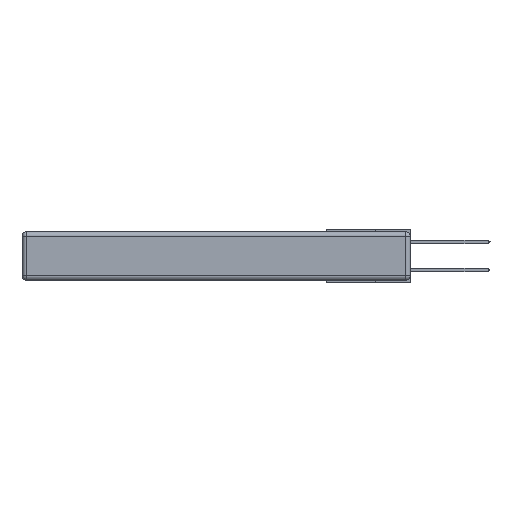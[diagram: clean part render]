
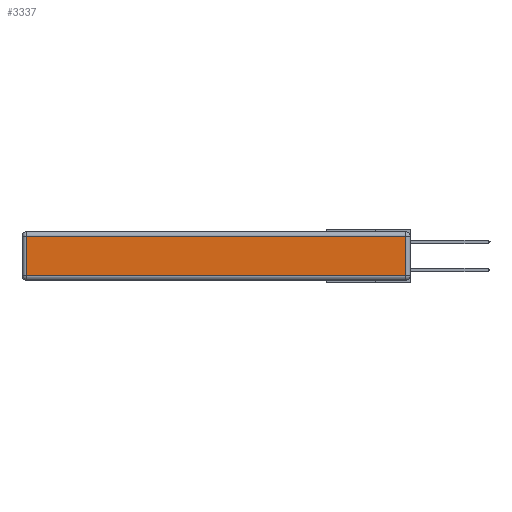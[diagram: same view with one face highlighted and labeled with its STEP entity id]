
A CAD part, left-side view. The second image highlights one B-rep face of the part: STEP entity #3337.
In plain terms, the highlighted planar face has unit normal (-1, 0, 0).
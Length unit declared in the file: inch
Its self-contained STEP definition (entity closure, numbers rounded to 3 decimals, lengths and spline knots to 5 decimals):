
#512 = VECTOR ( 'NONE', #9564, 39.37008 ) ;
#1010 = ORIENTED_EDGE ( 'NONE', *, *, #21946, .T. ) ;
#1089 = EDGE_CURVE ( 'NONE', #18587, #13305, #20870, .T. ) ;
#1495 = PLANE ( 'NONE',  #15933 ) ;
#1499 = DIRECTION ( 'NONE',  ( 0., 0., -1. ) ) ;
#2366 = CARTESIAN_POINT ( 'NONE',  ( 0., 2.75, -0.03 ) ) ;
#3337 = ADVANCED_FACE ( 'NONE', ( #21663 ), #1495, .T. ) ;
#3548 = DIRECTION ( 'NONE',  ( -1., 0., 0. ) ) ;
#3764 = ORIENTED_EDGE ( 'NONE', *, *, #1089, .T. ) ;
#4328 = CARTESIAN_POINT ( 'NONE',  ( 0., 0.03, -0.343 ) ) ;
#5006 = VERTEX_POINT ( 'NONE', #21774 ) ;
#8549 = VECTOR ( 'NONE', #8714, 39.37008 ) ;
#8714 = DIRECTION ( 'NONE',  ( 0., 1., 0. ) ) ;
#9564 = DIRECTION ( 'NONE',  ( 0., -1., 0. ) ) ;
#10054 = LINE ( 'NONE', #4328, #18641 ) ;
#10181 = EDGE_LOOP ( 'NONE', ( #3764, #17243, #1010, #20148 ) ) ;
#11650 = VECTOR ( 'NONE', #1499, 39.37008 ) ;
#13305 = VERTEX_POINT ( 'NONE', #22958 ) ;
#15309 = VERTEX_POINT ( 'NONE', #18770 ) ;
#15757 = CARTESIAN_POINT ( 'NONE',  ( 0., 0., -0.343 ) ) ;
#15778 = CARTESIAN_POINT ( 'NONE',  ( 0., 0., -0.313 ) ) ;
#15933 = AXIS2_PLACEMENT_3D ( 'NONE', #15757, #3548, #17799 ) ;
#16282 = EDGE_CURVE ( 'NONE', #5006, #18587, #18327, .T. ) ;
#17243 = ORIENTED_EDGE ( 'NONE', *, *, #23346, .T. ) ;
#17799 = DIRECTION ( 'NONE',  ( 0., 0., 1. ) ) ;
#18327 = LINE ( 'NONE', #21660, #11650 ) ;
#18587 = VERTEX_POINT ( 'NONE', #21472 ) ;
#18641 = VECTOR ( 'NONE', #24907, 39.37008 ) ;
#18770 = CARTESIAN_POINT ( 'NONE',  ( 0., 0.03, -0.03 ) ) ;
#19332 = LINE ( 'NONE', #2366, #8549 ) ;
#20148 = ORIENTED_EDGE ( 'NONE', *, *, #16282, .T. ) ;
#20870 = LINE ( 'NONE', #15778, #512 ) ;
#21472 = CARTESIAN_POINT ( 'NONE',  ( 0., 2.72, -0.313 ) ) ;
#21660 = CARTESIAN_POINT ( 'NONE',  ( 0., 2.72, -0.343 ) ) ;
#21663 = FACE_OUTER_BOUND ( 'NONE', #10181, .T. ) ;
#21774 = CARTESIAN_POINT ( 'NONE',  ( 0., 2.72, -0.03 ) ) ;
#21946 = EDGE_CURVE ( 'NONE', #15309, #5006, #19332, .T. ) ;
#22958 = CARTESIAN_POINT ( 'NONE',  ( 0., 0.03, -0.313 ) ) ;
#23346 = EDGE_CURVE ( 'NONE', #13305, #15309, #10054, .T. ) ;
#24907 = DIRECTION ( 'NONE',  ( 0., 0., 1. ) ) ;
